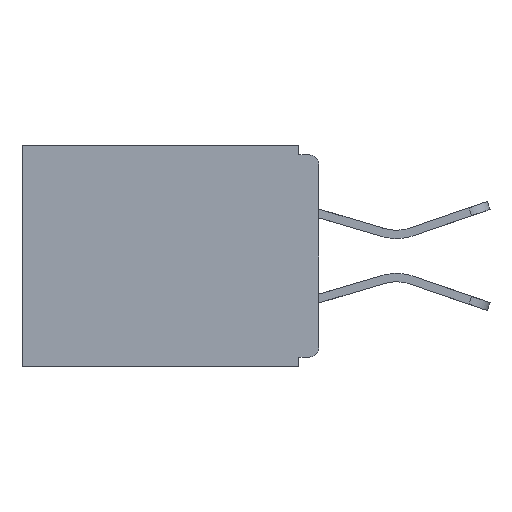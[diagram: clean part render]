
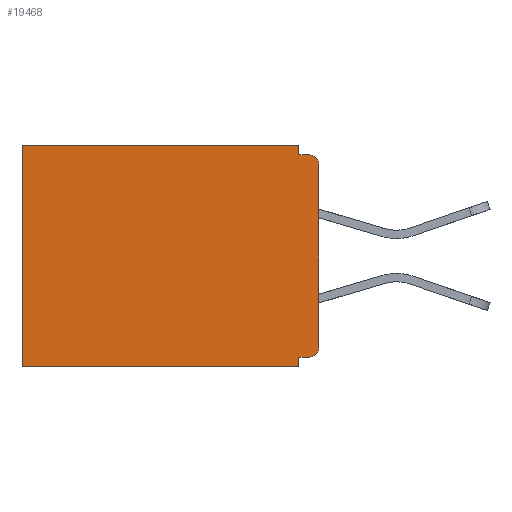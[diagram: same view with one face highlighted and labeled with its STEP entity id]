
A CAD part, left-side view. The second image highlights one B-rep face of the part: STEP entity #19468.
In plain terms, the highlighted planar face has unit normal (-1, 0, 0).
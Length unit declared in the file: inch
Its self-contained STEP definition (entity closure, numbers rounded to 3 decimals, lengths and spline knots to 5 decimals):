
#256 = EDGE_CURVE ( 'NONE', #21678, #922, #22315, .T. ) ;
#773 = AXIS2_PLACEMENT_3D ( 'NONE', #5181, #7083, #1547 ) ;
#781 = FACE_OUTER_BOUND ( 'NONE', #12631, .T. ) ;
#856 = VECTOR ( 'NONE', #22965, 39.37008 ) ;
#922 = VERTEX_POINT ( 'NONE', #23498 ) ;
#1209 = CARTESIAN_POINT ( 'NONE',  ( 0.298, 0., -0.328 ) ) ;
#1547 = DIRECTION ( 'NONE',  ( 0., 0., -1. ) ) ;
#2841 = VERTEX_POINT ( 'NONE', #8259 ) ;
#3074 = LINE ( 'NONE', #9244, #9642 ) ;
#3448 = LINE ( 'NONE', #16149, #20112 ) ;
#3510 = VECTOR ( 'NONE', #8748, 39.37008 ) ;
#3601 = VERTEX_POINT ( 'NONE', #10869 ) ;
#3693 = CARTESIAN_POINT ( 'NONE',  ( 0.298, 0.031, -0.343 ) ) ;
#4019 = ORIENTED_EDGE ( 'NONE', *, *, #5256, .F. ) ;
#4344 = LINE ( 'NONE', #14973, #18914 ) ;
#4534 = CIRCLE ( 'NONE', #23749, 0.015 ) ;
#4826 = EDGE_CURVE ( 'NONE', #2841, #15046, #3074, .T. ) ;
#5000 = DIRECTION ( 'NONE',  ( 0., 1., 0. ) ) ;
#5181 = CARTESIAN_POINT ( 'NONE',  ( 0.298, 0., 0. ) ) ;
#5256 = EDGE_CURVE ( 'NONE', #922, #3601, #12312, .T. ) ;
#5519 = CARTESIAN_POINT ( 'NONE',  ( 0.298, 0.031, -0.015 ) ) ;
#5593 = CARTESIAN_POINT ( 'NONE',  ( 0.298, 0.031, 0. ) ) ;
#5761 = ORIENTED_EDGE ( 'NONE', *, *, #7871, .T. ) ;
#5909 = EDGE_CURVE ( 'NONE', #9122, #18867, #24170, .T. ) ;
#6531 = VECTOR ( 'NONE', #17250, 39.37008 ) ;
#6651 = AXIS2_PLACEMENT_3D ( 'NONE', #14054, #6716, #23864 ) ;
#6716 = DIRECTION ( 'NONE',  ( -1., 0., 0. ) ) ;
#6837 = EDGE_CURVE ( 'NONE', #2841, #14191, #16099, .T. ) ;
#7083 = DIRECTION ( 'NONE',  ( 1., 0., 0. ) ) ;
#7377 = DIRECTION ( 'NONE',  ( 0., 0., -1. ) ) ;
#7871 = EDGE_CURVE ( 'NONE', #23739, #15046, #4534, .T. ) ;
#8259 = CARTESIAN_POINT ( 'NONE',  ( 0.298, 0., -0.03 ) ) ;
#8591 = LINE ( 'NONE', #1209, #3510 ) ;
#8727 = CARTESIAN_POINT ( 'NONE',  ( 0.298, 0.015, -0.015 ) ) ;
#8739 = ORIENTED_EDGE ( 'NONE', *, *, #256, .F. ) ;
#8748 = DIRECTION ( 'NONE',  ( 0., 1., 0. ) ) ;
#9122 = VERTEX_POINT ( 'NONE', #5593 ) ;
#9231 = ORIENTED_EDGE ( 'NONE', *, *, #5909, .T. ) ;
#9244 = CARTESIAN_POINT ( 'NONE',  ( 0.298, 0., 0. ) ) ;
#9642 = VECTOR ( 'NONE', #10990, 39.37008 ) ;
#9707 = CARTESIAN_POINT ( 'NONE',  ( 0.298, 0.015, -0.328 ) ) ;
#10510 = VECTOR ( 'NONE', #5000, 39.37008 ) ;
#10801 = DIRECTION ( 'NONE',  ( 0., -1., 0. ) ) ;
#10869 = CARTESIAN_POINT ( 'NONE',  ( 0.298, 0.46, -0.343 ) ) ;
#10990 = DIRECTION ( 'NONE',  ( 0., 0., -1. ) ) ;
#12014 = DIRECTION ( 'NONE',  ( 0., 0., -1. ) ) ;
#12312 = LINE ( 'NONE', #23817, #10510 ) ;
#12631 = EDGE_LOOP ( 'NONE', ( #17855, #15164, #21829, #9231, #13451, #4019, #8739, #22762, #5761, #23433 ) ) ;
#12856 = VECTOR ( 'NONE', #23401, 39.37008 ) ;
#13451 = ORIENTED_EDGE ( 'NONE', *, *, #24425, .T. ) ;
#14054 = CARTESIAN_POINT ( 'NONE',  ( 0.298, 0.015, -0.03 ) ) ;
#14191 = VERTEX_POINT ( 'NONE', #8727 ) ;
#14305 = EDGE_CURVE ( 'NONE', #22419, #14191, #3448, .T. ) ;
#14544 = EDGE_CURVE ( 'NONE', #9122, #22419, #4344, .T. ) ;
#14973 = CARTESIAN_POINT ( 'NONE',  ( 0.298, 0.031, -0.343 ) ) ;
#15046 = VERTEX_POINT ( 'NONE', #20264 ) ;
#15164 = ORIENTED_EDGE ( 'NONE', *, *, #14305, .F. ) ;
#15784 = LINE ( 'NONE', #19379, #856 ) ;
#16099 = CIRCLE ( 'NONE', #6651, 0.015 ) ;
#16149 = CARTESIAN_POINT ( 'NONE',  ( 0.298, 0., -0.015 ) ) ;
#16665 = CARTESIAN_POINT ( 'NONE',  ( 0.298, 0.46, 0. ) ) ;
#17250 = DIRECTION ( 'NONE',  ( 0., 0., -1. ) ) ;
#17855 = ORIENTED_EDGE ( 'NONE', *, *, #6837, .T. ) ;
#18867 = VERTEX_POINT ( 'NONE', #16665 ) ;
#18914 = VECTOR ( 'NONE', #7377, 39.37008 ) ;
#19379 = CARTESIAN_POINT ( 'NONE',  ( 0.298, 0.46, 0. ) ) ;
#19390 = EDGE_CURVE ( 'NONE', #23739, #21678, #8591, .T. ) ;
#19468 = ADVANCED_FACE ( 'NONE', ( #781 ), #22152, .F. ) ;
#20112 = VECTOR ( 'NONE', #10801, 39.37008 ) ;
#20264 = CARTESIAN_POINT ( 'NONE',  ( 0.298, 0., -0.313 ) ) ;
#20750 = CARTESIAN_POINT ( 'NONE',  ( 0.298, 0.031, -0.328 ) ) ;
#21476 = CARTESIAN_POINT ( 'NONE',  ( 0.298, 0.015, -0.313 ) ) ;
#21678 = VERTEX_POINT ( 'NONE', #20750 ) ;
#21829 = ORIENTED_EDGE ( 'NONE', *, *, #14544, .F. ) ;
#22152 = PLANE ( 'NONE',  #773 ) ;
#22315 = LINE ( 'NONE', #3693, #6531 ) ;
#22419 = VERTEX_POINT ( 'NONE', #5519 ) ;
#22762 = ORIENTED_EDGE ( 'NONE', *, *, #19390, .F. ) ;
#22965 = DIRECTION ( 'NONE',  ( 0., 0., -1. ) ) ;
#23325 = CARTESIAN_POINT ( 'NONE',  ( 0.298, 0., 0. ) ) ;
#23401 = DIRECTION ( 'NONE',  ( 0., 1., 0. ) ) ;
#23408 = DIRECTION ( 'NONE',  ( -1., 0., 0. ) ) ;
#23433 = ORIENTED_EDGE ( 'NONE', *, *, #4826, .F. ) ;
#23498 = CARTESIAN_POINT ( 'NONE',  ( 0.298, 0.031, -0.343 ) ) ;
#23739 = VERTEX_POINT ( 'NONE', #9707 ) ;
#23749 = AXIS2_PLACEMENT_3D ( 'NONE', #21476, #23408, #12014 ) ;
#23817 = CARTESIAN_POINT ( 'NONE',  ( 0.298, 0., -0.343 ) ) ;
#23864 = DIRECTION ( 'NONE',  ( 0., 0., -1. ) ) ;
#24170 = LINE ( 'NONE', #23325, #12856 ) ;
#24425 = EDGE_CURVE ( 'NONE', #18867, #3601, #15784, .T. ) ;
